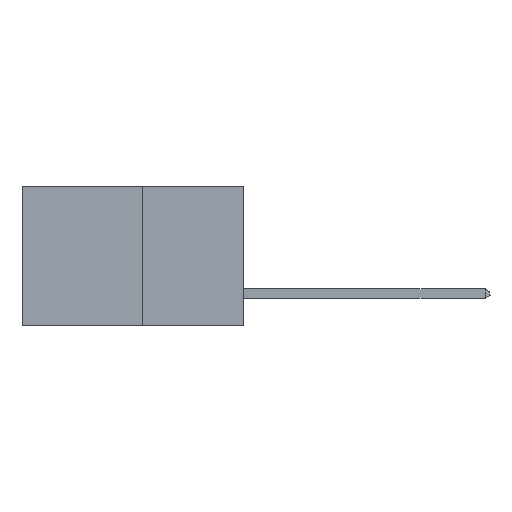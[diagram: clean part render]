
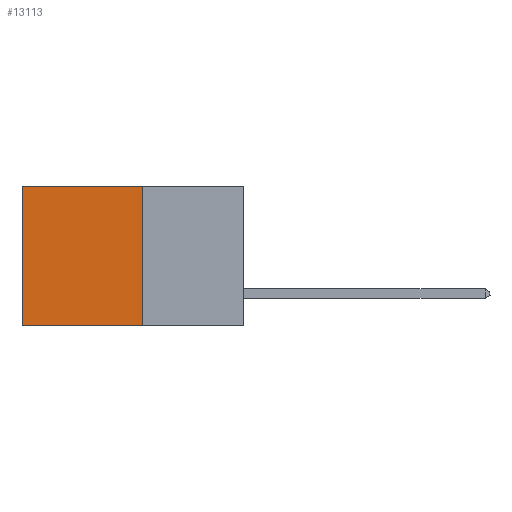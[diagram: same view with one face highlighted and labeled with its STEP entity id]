
A CAD part, left-side view. The second image highlights one B-rep face of the part: STEP entity #13113.
In plain terms, the highlighted planar face has unit normal (-1, 0, 0).
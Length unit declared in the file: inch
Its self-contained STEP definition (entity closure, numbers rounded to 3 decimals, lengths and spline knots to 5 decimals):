
#180 = ORIENTED_EDGE ( 'NONE', *, *, #22070, .F. ) ;
#338 = CARTESIAN_POINT ( 'NONE',  ( 0.277, 0.59, -0.37 ) ) ;
#1379 = LINE ( 'NONE', #27357, #23648 ) ;
#1981 = VERTEX_POINT ( 'NONE', #9533 ) ;
#2841 = LINE ( 'NONE', #4519, #19355 ) ;
#3610 = DIRECTION ( 'NONE',  ( 0., 1., 0. ) ) ;
#3982 = ORIENTED_EDGE ( 'NONE', *, *, #22374, .T. ) ;
#4519 = CARTESIAN_POINT ( 'NONE',  ( 0.277, 0.27, -0.37 ) ) ;
#4692 = DIRECTION ( 'NONE',  ( 0., 0., -1. ) ) ;
#4746 = LINE ( 'NONE', #338, #9789 ) ;
#6136 = ORIENTED_EDGE ( 'NONE', *, *, #8752, .T. ) ;
#6487 = EDGE_CURVE ( 'NONE', #8956, #1981, #2841, .T. ) ;
#6897 = PLANE ( 'NONE',  #15830 ) ;
#8752 = EDGE_CURVE ( 'NONE', #8956, #19528, #16915, .T. ) ;
#8956 = VERTEX_POINT ( 'NONE', #23686 ) ;
#8957 = CARTESIAN_POINT ( 'NONE',  ( 0.277, 0.27, -0.37 ) ) ;
#9128 = CARTESIAN_POINT ( 'NONE',  ( 0.277, 0.59, 0. ) ) ;
#9533 = CARTESIAN_POINT ( 'NONE',  ( 0.277, 0.27, -0.37 ) ) ;
#9789 = VECTOR ( 'NONE', #4692, 39.37008 ) ;
#9816 = VECTOR ( 'NONE', #3610, 39.37008 ) ;
#11211 = DIRECTION ( 'NONE',  ( 0., 0., -1. ) ) ;
#13113 = ADVANCED_FACE ( 'NONE', ( #19039 ), #6897, .F. ) ;
#14372 = CARTESIAN_POINT ( 'NONE',  ( 0.277, 0.27, 0. ) ) ;
#15830 = AXIS2_PLACEMENT_3D ( 'NONE', #8957, #24147, #11211 ) ;
#16469 = CARTESIAN_POINT ( 'NONE',  ( 0.277, 0.59, -0.37 ) ) ;
#16915 = LINE ( 'NONE', #14372, #9816 ) ;
#17935 = VERTEX_POINT ( 'NONE', #16469 ) ;
#19039 = FACE_OUTER_BOUND ( 'NONE', #26589, .T. ) ;
#19355 = VECTOR ( 'NONE', #22203, 39.37008 ) ;
#19528 = VERTEX_POINT ( 'NONE', #9128 ) ;
#20918 = DIRECTION ( 'NONE',  ( 0., 1., 0. ) ) ;
#22070 = EDGE_CURVE ( 'NONE', #1981, #17935, #1379, .T. ) ;
#22203 = DIRECTION ( 'NONE',  ( 0., 0., -1. ) ) ;
#22374 = EDGE_CURVE ( 'NONE', #19528, #17935, #4746, .T. ) ;
#23648 = VECTOR ( 'NONE', #20918, 39.37008 ) ;
#23686 = CARTESIAN_POINT ( 'NONE',  ( 0.277, 0.27, 0. ) ) ;
#24147 = DIRECTION ( 'NONE',  ( 1., 0., 0. ) ) ;
#26589 = EDGE_LOOP ( 'NONE', ( #3982, #180, #27169, #6136 ) ) ;
#27169 = ORIENTED_EDGE ( 'NONE', *, *, #6487, .F. ) ;
#27357 = CARTESIAN_POINT ( 'NONE',  ( 0.277, 0.27, -0.37 ) ) ;
